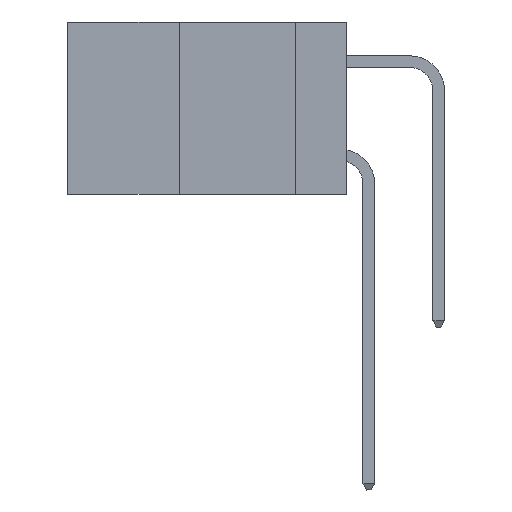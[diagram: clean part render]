
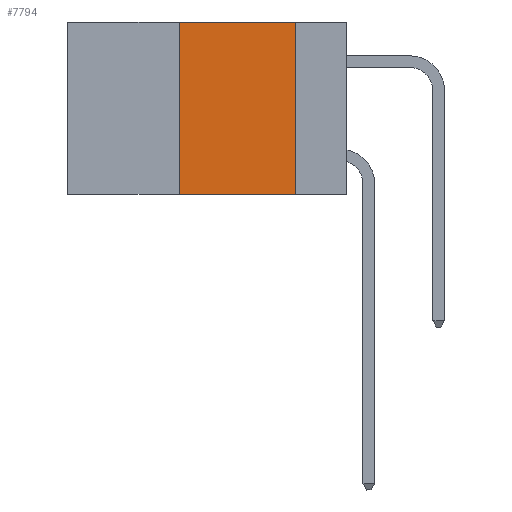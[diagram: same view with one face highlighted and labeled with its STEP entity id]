
A CAD part, left-side view. The second image highlights one B-rep face of the part: STEP entity #7794.
In plain terms, the highlighted planar face has unit normal (-1, 0, 0).
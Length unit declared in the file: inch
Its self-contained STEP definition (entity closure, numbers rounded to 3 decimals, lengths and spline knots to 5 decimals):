
#566 = AXIS2_PLACEMENT_3D ( 'NONE', #5146, #27395, #8368 ) ;
#620 = VECTOR ( 'NONE', #40178, 39.37008 ) ;
#1135 = VERTEX_POINT ( 'NONE', #18386 ) ;
#2808 = LINE ( 'NONE', #2936, #27241 ) ;
#2936 = CARTESIAN_POINT ( 'NONE',  ( 0., 0.11, 0. ) ) ;
#2969 = VERTEX_POINT ( 'NONE', #40586 ) ;
#3191 = DIRECTION ( 'NONE',  ( 0., 0., 1. ) ) ;
#5146 = CARTESIAN_POINT ( 'NONE',  ( 0., 0.6, 0. ) ) ;
#7794 = ADVANCED_FACE ( 'NONE', ( #8845 ), #36762, .F. ) ;
#8368 = DIRECTION ( 'NONE',  ( 0., 0., -1. ) ) ;
#8845 = FACE_OUTER_BOUND ( 'NONE', #9523, .T. ) ;
#9523 = EDGE_LOOP ( 'NONE', ( #12333, #37557, #14299, #19310 ) ) ;
#11750 = CARTESIAN_POINT ( 'NONE',  ( 0., 0.6, -0.37 ) ) ;
#12333 = ORIENTED_EDGE ( 'NONE', *, *, #29056, .F. ) ;
#14299 = ORIENTED_EDGE ( 'NONE', *, *, #35398, .F. ) ;
#17035 = CARTESIAN_POINT ( 'NONE',  ( 0., 0.11, 0. ) ) ;
#18386 = CARTESIAN_POINT ( 'NONE',  ( 0., 0.11, -0.37 ) ) ;
#18711 = LINE ( 'NONE', #11750, #620 ) ;
#19310 = ORIENTED_EDGE ( 'NONE', *, *, #19768, .T. ) ;
#19768 = EDGE_CURVE ( 'NONE', #32918, #1135, #18711, .T. ) ;
#24183 = VECTOR ( 'NONE', #3191, 39.37008 ) ;
#25600 = CARTESIAN_POINT ( 'NONE',  ( 0., 0.6, 0. ) ) ;
#27241 = VECTOR ( 'NONE', #37766, 39.37008 ) ;
#27395 = DIRECTION ( 'NONE',  ( 1., 0., 0. ) ) ;
#28458 = LINE ( 'NONE', #25600, #34885 ) ;
#28808 = DIRECTION ( 'NONE',  ( 0., -1., 0. ) ) ;
#29056 = EDGE_CURVE ( 'NONE', #39937, #1135, #2808, .T. ) ;
#29482 = CARTESIAN_POINT ( 'NONE',  ( 0., 0.36, -0.37 ) ) ;
#32628 = LINE ( 'NONE', #41120, #24183 ) ;
#32918 = VERTEX_POINT ( 'NONE', #29482 ) ;
#34885 = VECTOR ( 'NONE', #28808, 39.37008 ) ;
#35398 = EDGE_CURVE ( 'NONE', #32918, #2969, #32628, .T. ) ;
#36762 = PLANE ( 'NONE',  #566 ) ;
#37557 = ORIENTED_EDGE ( 'NONE', *, *, #38423, .F. ) ;
#37766 = DIRECTION ( 'NONE',  ( 0., 0., -1. ) ) ;
#38423 = EDGE_CURVE ( 'NONE', #2969, #39937, #28458, .T. ) ;
#39937 = VERTEX_POINT ( 'NONE', #17035 ) ;
#40178 = DIRECTION ( 'NONE',  ( 0., -1., 0. ) ) ;
#40586 = CARTESIAN_POINT ( 'NONE',  ( 0., 0.36, 0. ) ) ;
#41120 = CARTESIAN_POINT ( 'NONE',  ( 0., 0.36, 0. ) ) ;
